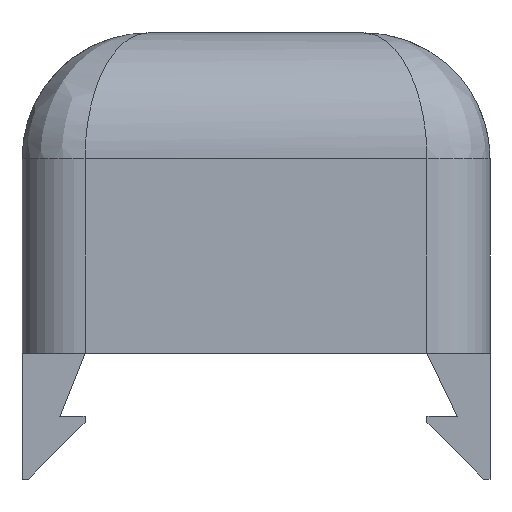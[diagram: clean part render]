
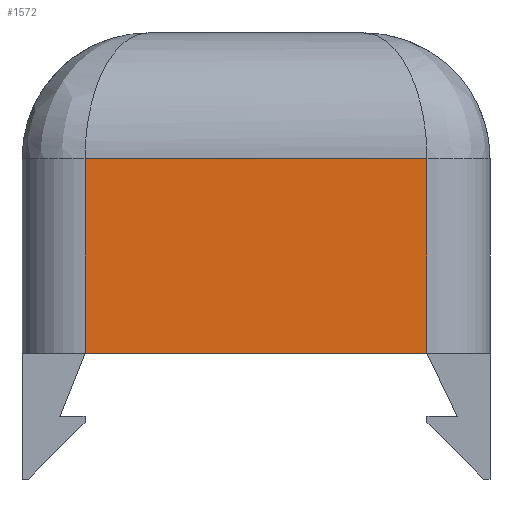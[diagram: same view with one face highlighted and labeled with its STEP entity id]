
A CAD part, front view. The second image highlights one B-rep face of the part: STEP entity #1572.
In plain terms, the highlighted planar face has unit normal (0, -1, 0).
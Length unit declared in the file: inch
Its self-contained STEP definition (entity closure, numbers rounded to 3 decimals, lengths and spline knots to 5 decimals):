
#145 = LINE ( 'NONE', #1148, #1073 ) ;
#168 = EDGE_CURVE ( 'NONE', #1253, #243, #521, .T. ) ;
#190 = VECTOR ( 'NONE', #1536, 39.37008 ) ;
#243 = VERTEX_POINT ( 'NONE', #586 ) ;
#266 = DIRECTION ( 'NONE',  ( 1., 0., 0. ) ) ;
#300 = DIRECTION ( 'NONE',  ( 0., 0., -1. ) ) ;
#363 = CARTESIAN_POINT ( 'NONE',  ( -0.57117, -2.04944, 0.6063 ) ) ;
#419 = VECTOR ( 'NONE', #266, 39.37008 ) ;
#430 = PLANE ( 'NONE',  #948 ) ;
#439 = EDGE_LOOP ( 'NONE', ( #1343, #1095, #534, #529 ) ) ;
#478 = VECTOR ( 'NONE', #300, 39.37008 ) ;
#497 = EDGE_CURVE ( 'NONE', #1039, #940, #806, .T. ) ;
#498 = LINE ( 'NONE', #1396, #419 ) ;
#518 = DIRECTION ( 'NONE',  ( -1., 0., 0. ) ) ;
#521 = LINE ( 'NONE', #1157, #190 ) ;
#529 = ORIENTED_EDGE ( 'NONE', *, *, #1425, .T. ) ;
#534 = ORIENTED_EDGE ( 'NONE', *, *, #168, .T. ) ;
#586 = CARTESIAN_POINT ( 'NONE',  ( -0.57117, -2.04944, 0. ) ) ;
#675 = DIRECTION ( 'NONE',  ( 0., 1., 0. ) ) ;
#794 = CARTESIAN_POINT ( 'NONE',  ( 0.49707, -2.04944, 0.6063 ) ) ;
#806 = LINE ( 'NONE', #1185, #478 ) ;
#918 = EDGE_CURVE ( 'NONE', #1039, #1253, #145, .T. ) ;
#940 = VERTEX_POINT ( 'NONE', #1277 ) ;
#948 = AXIS2_PLACEMENT_3D ( 'NONE', #1311, #675, #1558 ) ;
#1039 = VERTEX_POINT ( 'NONE', #794 ) ;
#1073 = VECTOR ( 'NONE', #518, 39.37008 ) ;
#1095 = ORIENTED_EDGE ( 'NONE', *, *, #918, .T. ) ;
#1148 = CARTESIAN_POINT ( 'NONE',  ( -0.57117, -2.04944, 0.6063 ) ) ;
#1157 = CARTESIAN_POINT ( 'NONE',  ( -0.57117, -2.04944, 0.03937 ) ) ;
#1185 = CARTESIAN_POINT ( 'NONE',  ( 0.49707, -2.04944, 0.03937 ) ) ;
#1253 = VERTEX_POINT ( 'NONE', #363 ) ;
#1277 = CARTESIAN_POINT ( 'NONE',  ( 0.49707, -2.04944, 0. ) ) ;
#1311 = CARTESIAN_POINT ( 'NONE',  ( -0.57117, -2.04944, 0.03937 ) ) ;
#1343 = ORIENTED_EDGE ( 'NONE', *, *, #497, .F. ) ;
#1395 = FACE_OUTER_BOUND ( 'NONE', #439, .T. ) ;
#1396 = CARTESIAN_POINT ( 'NONE',  ( -0.57117, -2.04944, 0. ) ) ;
#1425 = EDGE_CURVE ( 'NONE', #243, #940, #498, .T. ) ;
#1536 = DIRECTION ( 'NONE',  ( 0., 0., -1. ) ) ;
#1558 = DIRECTION ( 'NONE',  ( 0., 0., 1. ) ) ;
#1572 = ADVANCED_FACE ( 'NONE', ( #1395 ), #430, .F. ) ;
